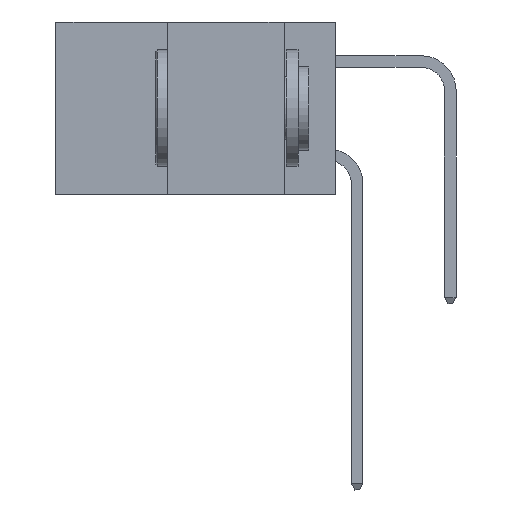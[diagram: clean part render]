
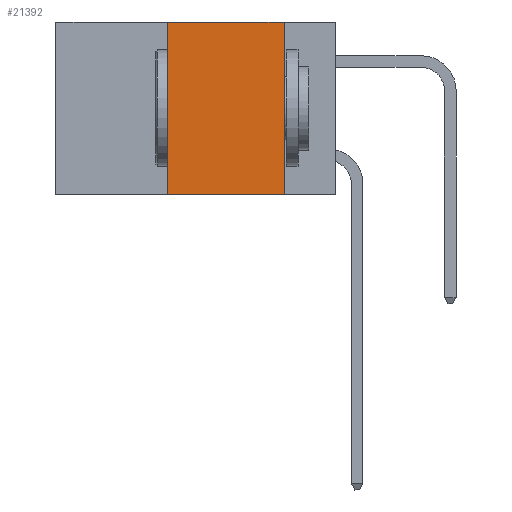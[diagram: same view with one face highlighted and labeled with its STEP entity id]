
A CAD part, left-side view. The second image highlights one B-rep face of the part: STEP entity #21392.
In plain terms, the highlighted planar face has unit normal (-1, 0, 0).
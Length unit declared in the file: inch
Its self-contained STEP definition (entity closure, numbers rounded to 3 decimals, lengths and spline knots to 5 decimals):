
#485 = CARTESIAN_POINT ( 'NONE',  ( 0., 0.6, 0. ) ) ;
#1074 = CARTESIAN_POINT ( 'NONE',  ( 0., 0.11, 0. ) ) ;
#1418 = VECTOR ( 'NONE', #17498, 39.37008 ) ;
#4283 = DIRECTION ( 'NONE',  ( 0., 0., 1. ) ) ;
#5790 = VECTOR ( 'NONE', #4283, 39.37008 ) ;
#5797 = CARTESIAN_POINT ( 'NONE',  ( 0., 0.11, 0. ) ) ;
#7521 = VECTOR ( 'NONE', #14158, 39.37008 ) ;
#8279 = CARTESIAN_POINT ( 'NONE',  ( 0., 0.6, 0. ) ) ;
#8333 = ORIENTED_EDGE ( 'NONE', *, *, #10579, .F. ) ;
#8339 = CARTESIAN_POINT ( 'NONE',  ( 0., 0.36, 0. ) ) ;
#9202 = VERTEX_POINT ( 'NONE', #13165 ) ;
#9527 = VERTEX_POINT ( 'NONE', #8339 ) ;
#9541 = FACE_OUTER_BOUND ( 'NONE', #11274, .T. ) ;
#9754 = VERTEX_POINT ( 'NONE', #1074 ) ;
#10211 = DIRECTION ( 'NONE',  ( 0., 0., -1. ) ) ;
#10579 = EDGE_CURVE ( 'NONE', #9754, #15203, #11905, .T. ) ;
#11274 = EDGE_LOOP ( 'NONE', ( #8333, #22746, #20993, #24780 ) ) ;
#11599 = DIRECTION ( 'NONE',  ( 0., 0., -1. ) ) ;
#11905 = LINE ( 'NONE', #5797, #16395 ) ;
#13165 = CARTESIAN_POINT ( 'NONE',  ( 0., 0.36, -0.37 ) ) ;
#14158 = DIRECTION ( 'NONE',  ( 0., -1., 0. ) ) ;
#15203 = VERTEX_POINT ( 'NONE', #18353 ) ;
#15936 = CARTESIAN_POINT ( 'NONE',  ( 0., 0.36, 0. ) ) ;
#16395 = VECTOR ( 'NONE', #11599, 39.37008 ) ;
#16919 = LINE ( 'NONE', #19374, #1418 ) ;
#17472 = EDGE_CURVE ( 'NONE', #9202, #15203, #16919, .T. ) ;
#17498 = DIRECTION ( 'NONE',  ( 0., -1., 0. ) ) ;
#17728 = LINE ( 'NONE', #485, #7521 ) ;
#18353 = CARTESIAN_POINT ( 'NONE',  ( 0., 0.11, -0.37 ) ) ;
#18946 = EDGE_CURVE ( 'NONE', #9527, #9754, #17728, .T. ) ;
#19329 = AXIS2_PLACEMENT_3D ( 'NONE', #8279, #21595, #10211 ) ;
#19374 = CARTESIAN_POINT ( 'NONE',  ( 0., 0.6, -0.37 ) ) ;
#19710 = PLANE ( 'NONE',  #19329 ) ;
#20495 = LINE ( 'NONE', #15936, #5790 ) ;
#20993 = ORIENTED_EDGE ( 'NONE', *, *, #24539, .F. ) ;
#21392 = ADVANCED_FACE ( 'NONE', ( #9541 ), #19710, .F. ) ;
#21595 = DIRECTION ( 'NONE',  ( 1., 0., 0. ) ) ;
#22746 = ORIENTED_EDGE ( 'NONE', *, *, #18946, .F. ) ;
#24539 = EDGE_CURVE ( 'NONE', #9202, #9527, #20495, .T. ) ;
#24780 = ORIENTED_EDGE ( 'NONE', *, *, #17472, .T. ) ;
